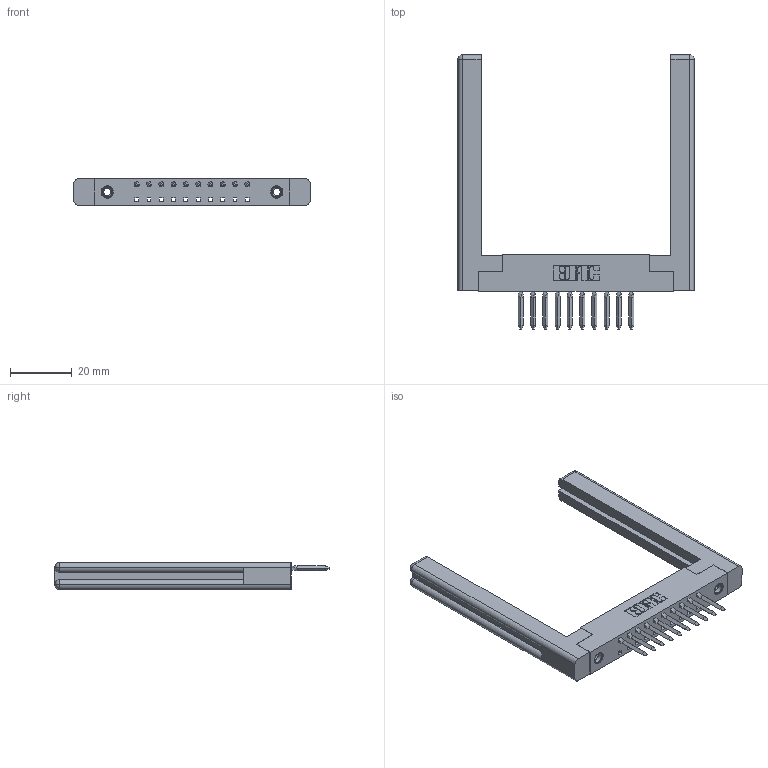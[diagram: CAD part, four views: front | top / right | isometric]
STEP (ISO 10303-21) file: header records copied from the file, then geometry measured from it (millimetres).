
FILE_DESCRIPTION (( 'STEP AP203' ), '1' );
FILE_NAME ('338-010-540-178.STEP', '2020-03-24T16:53:03', ( '' ), ( '' ), 'SwSTEP 2.0', 'SolidWorks 2016', '' );
FILE_SCHEMA (( 'CONFIG_CONTROL_DESIGN' ));
Length unit declared in the file: inch
Products named in the file (5): 307-220-058; 345-250-001_345-250-001-102; 338-210-001_338-210-010-004; 338-290-001_540; 338-010-540-178
Assembly tree (15 placements, depth 2):
  338-010-540-178
    338-210-001_338-210-010-004
    338-290-001_540  x10
    345-250-001_345-250-001-102  x2
    307-220-058  x2
Bounding box: 76.25 x 88.52 x 8.71 mm (x, y, z)
Volume: 12830.9 mm3; surface area: 12838.6 mm2
Topology: 15 solids, 15 shells, 1166 faces, 3175 edges, 2030 vertices
Faces by surface type: plane 784, cylinder 318, bspline 40, cone 12, torus 12
Entity records: 25237 total; most frequent: CARTESIAN_POINT 5065, ORIENTED_EDGE 4178, DIRECTION 3916, EDGE_CURVE 2089, LINE 1510, VECTOR 1510, VERTEX_POINT 1354, AXIS2_PLACEMENT_3D 1203
